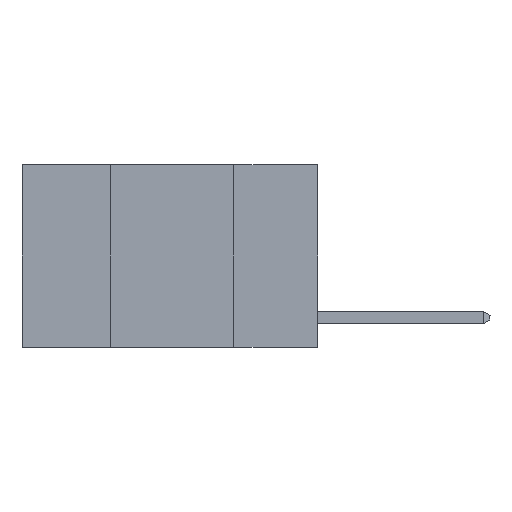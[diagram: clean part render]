
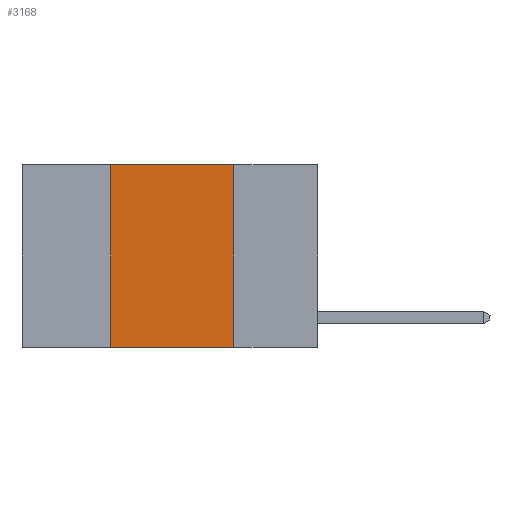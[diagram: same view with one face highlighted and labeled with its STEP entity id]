
A CAD part, left-side view. The second image highlights one B-rep face of the part: STEP entity #3168.
In plain terms, the highlighted planar face has unit normal (-1, 0, 0).
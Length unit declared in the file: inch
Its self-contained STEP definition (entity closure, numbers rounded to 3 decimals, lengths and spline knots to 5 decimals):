
#346 = VERTEX_POINT ( 'NONE', #13249 ) ;
#1186 = ORIENTED_EDGE ( 'NONE', *, *, #8525, .F. ) ;
#1364 = CARTESIAN_POINT ( 'NONE',  ( 0., 0.6, 0. ) ) ;
#2144 = LINE ( 'NONE', #3507, #10311 ) ;
#2310 = AXIS2_PLACEMENT_3D ( 'NONE', #1364, #2489, #7085 ) ;
#2385 = CARTESIAN_POINT ( 'NONE',  ( 0., 0.42, 0. ) ) ;
#2489 = DIRECTION ( 'NONE',  ( 1., 0., 0. ) ) ;
#3168 = ADVANCED_FACE ( 'NONE', ( #12852 ), #10076, .F. ) ;
#3406 = EDGE_CURVE ( 'NONE', #3559, #346, #12077, .T. ) ;
#3507 = CARTESIAN_POINT ( 'NONE',  ( 0., 0.6, -0.37 ) ) ;
#3559 = VERTEX_POINT ( 'NONE', #13108 ) ;
#3693 = ORIENTED_EDGE ( 'NONE', *, *, #14149, .F. ) ;
#4160 = DIRECTION ( 'NONE',  ( 0., -1., 0. ) ) ;
#4540 = EDGE_LOOP ( 'NONE', ( #9758, #1186, #3693, #10290 ) ) ;
#4573 = DIRECTION ( 'NONE',  ( 0., -1., 0. ) ) ;
#5337 = CARTESIAN_POINT ( 'NONE',  ( 0., 0.6, 0. ) ) ;
#6544 = DIRECTION ( 'NONE',  ( 0., 0., -1. ) ) ;
#6643 = VECTOR ( 'NONE', #6544, 39.37008 ) ;
#7085 = DIRECTION ( 'NONE',  ( 0., 0., -1. ) ) ;
#8525 = EDGE_CURVE ( 'NONE', #14356, #3559, #10944, .T. ) ;
#8738 = LINE ( 'NONE', #12315, #10784 ) ;
#9758 = ORIENTED_EDGE ( 'NONE', *, *, #3406, .F. ) ;
#10076 = PLANE ( 'NONE',  #2310 ) ;
#10290 = ORIENTED_EDGE ( 'NONE', *, *, #14716, .T. ) ;
#10311 = VECTOR ( 'NONE', #4573, 39.37008 ) ;
#10784 = VECTOR ( 'NONE', #13359, 39.37008 ) ;
#10944 = LINE ( 'NONE', #5337, #12706 ) ;
#11164 = VERTEX_POINT ( 'NONE', #14448 ) ;
#12077 = LINE ( 'NONE', #12310, #6643 ) ;
#12310 = CARTESIAN_POINT ( 'NONE',  ( 0., 0.17, 0. ) ) ;
#12315 = CARTESIAN_POINT ( 'NONE',  ( 0., 0.42, 0. ) ) ;
#12706 = VECTOR ( 'NONE', #4160, 39.37008 ) ;
#12852 = FACE_OUTER_BOUND ( 'NONE', #4540, .T. ) ;
#13108 = CARTESIAN_POINT ( 'NONE',  ( 0., 0.17, 0. ) ) ;
#13249 = CARTESIAN_POINT ( 'NONE',  ( 0., 0.17, -0.37 ) ) ;
#13359 = DIRECTION ( 'NONE',  ( 0., 0., 1. ) ) ;
#14149 = EDGE_CURVE ( 'NONE', #11164, #14356, #8738, .T. ) ;
#14356 = VERTEX_POINT ( 'NONE', #2385 ) ;
#14448 = CARTESIAN_POINT ( 'NONE',  ( 0., 0.42, -0.37 ) ) ;
#14716 = EDGE_CURVE ( 'NONE', #11164, #346, #2144, .T. ) ;
